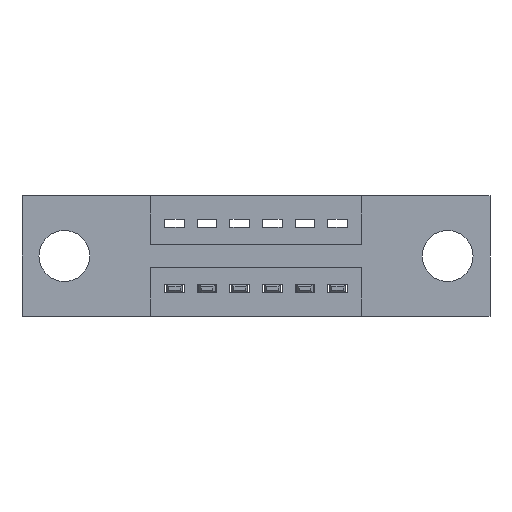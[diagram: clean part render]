
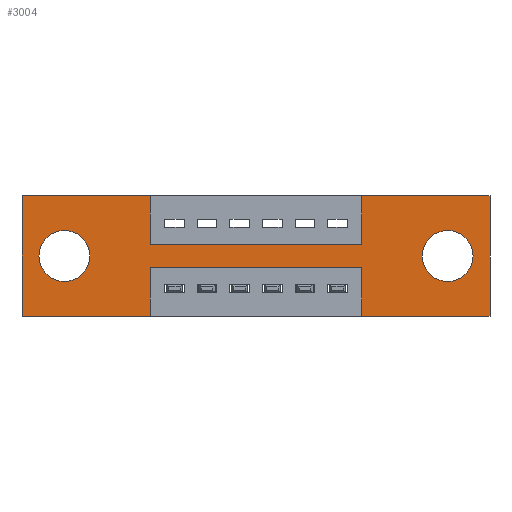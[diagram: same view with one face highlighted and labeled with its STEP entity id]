
A CAD part, front view. The second image highlights one B-rep face of the part: STEP entity #3004.
In plain terms, the highlighted planar face has unit normal (0, -1, 0).
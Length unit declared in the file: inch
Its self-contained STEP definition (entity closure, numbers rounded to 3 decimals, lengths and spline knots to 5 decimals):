
#263 = LINE ( 'NONE', #8894, #2155 ) ;
#273 = CARTESIAN_POINT ( 'NONE',  ( 0.13, 0., -0.185 ) ) ;
#449 = ORIENTED_EDGE ( 'NONE', *, *, #6010, .F. ) ;
#510 = ORIENTED_EDGE ( 'NONE', *, *, #3561, .F. ) ;
#656 = CARTESIAN_POINT ( 'NONE',  ( 0., 0., -0.37 ) ) ;
#702 = DIRECTION ( 'NONE',  ( 0., 0., 1. ) ) ;
#731 = CARTESIAN_POINT ( 'NONE',  ( 1.305, 0., -0.185 ) ) ;
#839 = AXIS2_PLACEMENT_3D ( 'NONE', #273, #4468, #7327 ) ;
#917 = EDGE_CURVE ( 'NONE', #7012, #8329, #1780, .T. ) ;
#924 = LINE ( 'NONE', #656, #3351 ) ;
#969 = FACE_BOUND ( 'NONE', #3698, .T. ) ;
#1025 = ORIENTED_EDGE ( 'NONE', *, *, #6048, .F. ) ;
#1088 = VECTOR ( 'NONE', #5413, 39.37008 ) ;
#1131 = ORIENTED_EDGE ( 'NONE', *, *, #6617, .F. ) ;
#1384 = CARTESIAN_POINT ( 'NONE',  ( 0.3925, 0., -0.22 ) ) ;
#1417 = EDGE_CURVE ( 'NONE', #2836, #5305, #6530, .T. ) ;
#1421 = LINE ( 'NONE', #6382, #8952 ) ;
#1458 = DIRECTION ( 'NONE',  ( -1., 0., 0. ) ) ;
#1647 = CARTESIAN_POINT ( 'NONE',  ( 0.13, 0., -0.263 ) ) ;
#1678 = EDGE_CURVE ( 'NONE', #3209, #7012, #3873, .T. ) ;
#1683 = AXIS2_PLACEMENT_3D ( 'NONE', #5897, #7960, #3851 ) ;
#1780 = LINE ( 'NONE', #1913, #9081 ) ;
#1822 = EDGE_CURVE ( 'NONE', #7105, #2836, #8498, .T. ) ;
#1888 = AXIS2_PLACEMENT_3D ( 'NONE', #3961, #8211, #2530 ) ;
#1913 = CARTESIAN_POINT ( 'NONE',  ( 0.3925, 0., -0.37 ) ) ;
#1924 = AXIS2_PLACEMENT_3D ( 'NONE', #731, #2257, #4273 ) ;
#1944 = VECTOR ( 'NONE', #5935, 39.37008 ) ;
#1992 = EDGE_CURVE ( 'NONE', #6641, #8614, #2429, .T. ) ;
#1994 = CIRCLE ( 'NONE', #1888, 0.078 ) ;
#2011 = CARTESIAN_POINT ( 'NONE',  ( 0., 0., 0. ) ) ;
#2080 = DIRECTION ( 'NONE',  ( 0., 0., 1. ) ) ;
#2155 = VECTOR ( 'NONE', #5618, 39.37008 ) ;
#2207 = CARTESIAN_POINT ( 'NONE',  ( 1.0425, 0., -0.15 ) ) ;
#2257 = DIRECTION ( 'NONE',  ( 0., 1., 0. ) ) ;
#2269 = ORIENTED_EDGE ( 'NONE', *, *, #5813, .T. ) ;
#2362 = ORIENTED_EDGE ( 'NONE', *, *, #7032, .T. ) ;
#2400 = ORIENTED_EDGE ( 'NONE', *, *, #1678, .F. ) ;
#2429 = LINE ( 'NONE', #4110, #9052 ) ;
#2519 = CARTESIAN_POINT ( 'NONE',  ( 1.435, 0., 0. ) ) ;
#2530 = DIRECTION ( 'NONE',  ( 0., 0., -1. ) ) ;
#2575 = VERTEX_POINT ( 'NONE', #5011 ) ;
#2611 = VECTOR ( 'NONE', #8573, 39.37008 ) ;
#2644 = DIRECTION ( 'NONE',  ( 0., 0., -1. ) ) ;
#2649 = EDGE_CURVE ( 'NONE', #3778, #6943, #4633, .T. ) ;
#2684 = EDGE_LOOP ( 'NONE', ( #4541, #2362 ) ) ;
#2734 = DIRECTION ( 'NONE',  ( -1., 0., 0. ) ) ;
#2836 = VERTEX_POINT ( 'NONE', #7200 ) ;
#2890 = CARTESIAN_POINT ( 'NONE',  ( 0., 0., 0. ) ) ;
#2916 = VERTEX_POINT ( 'NONE', #3874 ) ;
#2931 = VERTEX_POINT ( 'NONE', #7302 ) ;
#2967 = EDGE_LOOP ( 'NONE', ( #9012, #2400, #6961, #1025, #6428, #6770, #449, #8671, #7054, #510, #5293, #1131 ) ) ;
#2971 = EDGE_CURVE ( 'NONE', #2931, #7101, #3755, .T. ) ;
#3004 = ADVANCED_FACE ( 'NONE', ( #969, #5977, #8613 ), #8026, .T. ) ;
#3106 = CARTESIAN_POINT ( 'NONE',  ( 0., 0., -0.37 ) ) ;
#3209 = VERTEX_POINT ( 'NONE', #5916 ) ;
#3249 = CARTESIAN_POINT ( 'NONE',  ( 0., 0., 0. ) ) ;
#3351 = VECTOR ( 'NONE', #1458, 39.37008 ) ;
#3402 = VECTOR ( 'NONE', #8855, 39.37008 ) ;
#3561 = EDGE_CURVE ( 'NONE', #6943, #4788, #4296, .T. ) ;
#3698 = EDGE_LOOP ( 'NONE', ( #2269, #8166 ) ) ;
#3734 = CARTESIAN_POINT ( 'NONE',  ( 0., 0., 0. ) ) ;
#3755 = CIRCLE ( 'NONE', #839, 0.078 ) ;
#3778 = VERTEX_POINT ( 'NONE', #3106 ) ;
#3807 = CARTESIAN_POINT ( 'NONE',  ( 1.0425, 0., -0.37 ) ) ;
#3823 = EDGE_CURVE ( 'NONE', #4788, #6641, #6928, .T. ) ;
#3851 = DIRECTION ( 'NONE',  ( 0., 0., -1. ) ) ;
#3873 = LINE ( 'NONE', #5941, #3402 ) ;
#3874 = CARTESIAN_POINT ( 'NONE',  ( 1.305, 0., -0.107 ) ) ;
#3961 = CARTESIAN_POINT ( 'NONE',  ( 1.305, 0., -0.185 ) ) ;
#4110 = CARTESIAN_POINT ( 'NONE',  ( 0.3925, 0., -0.15 ) ) ;
#4216 = DIRECTION ( 'NONE',  ( 1., 0., 0. ) ) ;
#4273 = DIRECTION ( 'NONE',  ( 0., 0., -1. ) ) ;
#4296 = LINE ( 'NONE', #3734, #8361 ) ;
#4468 = DIRECTION ( 'NONE',  ( 0., 1., 0. ) ) ;
#4514 = CARTESIAN_POINT ( 'NONE',  ( 0.3925, 0., 0. ) ) ;
#4541 = ORIENTED_EDGE ( 'NONE', *, *, #2971, .T. ) ;
#4633 = LINE ( 'NONE', #2890, #2611 ) ;
#4710 = DIRECTION ( 'NONE',  ( 1., 0., 0. ) ) ;
#4788 = VERTEX_POINT ( 'NONE', #7256 ) ;
#5011 = CARTESIAN_POINT ( 'NONE',  ( 1.305, 0., -0.263 ) ) ;
#5250 = CIRCLE ( 'NONE', #8087, 0.078 ) ;
#5293 = ORIENTED_EDGE ( 'NONE', *, *, #2649, .F. ) ;
#5305 = VERTEX_POINT ( 'NONE', #7739 ) ;
#5310 = CARTESIAN_POINT ( 'NONE',  ( 0., 0., -0.37 ) ) ;
#5322 = CARTESIAN_POINT ( 'NONE',  ( 0.3925, 0., -0.37 ) ) ;
#5413 = DIRECTION ( 'NONE',  ( 0., 0., -1. ) ) ;
#5618 = DIRECTION ( 'NONE',  ( 0., 0., 1. ) ) ;
#5683 = DIRECTION ( 'NONE',  ( 0., 1., 0. ) ) ;
#5798 = VECTOR ( 'NONE', #2734, 39.37008 ) ;
#5813 = EDGE_CURVE ( 'NONE', #2916, #2575, #8559, .T. ) ;
#5897 = CARTESIAN_POINT ( 'NONE',  ( 0., 0., -0.37 ) ) ;
#5916 = CARTESIAN_POINT ( 'NONE',  ( 1.0425, 0., -0.22 ) ) ;
#5935 = DIRECTION ( 'NONE',  ( 0., 0., -1. ) ) ;
#5941 = CARTESIAN_POINT ( 'NONE',  ( 0.3925, 0., -0.22 ) ) ;
#5977 = FACE_BOUND ( 'NONE', #2684, .T. ) ;
#6010 = EDGE_CURVE ( 'NONE', #8614, #7105, #263, .T. ) ;
#6048 = EDGE_CURVE ( 'NONE', #5305, #9034, #924, .T. ) ;
#6322 = CARTESIAN_POINT ( 'NONE',  ( 0.13, 0., -0.185 ) ) ;
#6382 = CARTESIAN_POINT ( 'NONE',  ( 1.0425, 0., -0.37 ) ) ;
#6428 = ORIENTED_EDGE ( 'NONE', *, *, #1417, .F. ) ;
#6514 = CARTESIAN_POINT ( 'NONE',  ( 1.0425, 0., 0. ) ) ;
#6530 = LINE ( 'NONE', #2519, #1088 ) ;
#6551 = DIRECTION ( 'NONE',  ( 1., 0., 0. ) ) ;
#6617 = EDGE_CURVE ( 'NONE', #8329, #3778, #8429, .T. ) ;
#6641 = VERTEX_POINT ( 'NONE', #8870 ) ;
#6770 = ORIENTED_EDGE ( 'NONE', *, *, #1822, .F. ) ;
#6928 = LINE ( 'NONE', #4514, #1944 ) ;
#6943 = VERTEX_POINT ( 'NONE', #2011 ) ;
#6961 = ORIENTED_EDGE ( 'NONE', *, *, #8519, .F. ) ;
#7012 = VERTEX_POINT ( 'NONE', #1384 ) ;
#7032 = EDGE_CURVE ( 'NONE', #7101, #2931, #5250, .T. ) ;
#7054 = ORIENTED_EDGE ( 'NONE', *, *, #3823, .F. ) ;
#7101 = VERTEX_POINT ( 'NONE', #1647 ) ;
#7105 = VERTEX_POINT ( 'NONE', #6514 ) ;
#7200 = CARTESIAN_POINT ( 'NONE',  ( 1.435, 0., 0. ) ) ;
#7256 = CARTESIAN_POINT ( 'NONE',  ( 0.3925, 0., 0. ) ) ;
#7302 = CARTESIAN_POINT ( 'NONE',  ( 0.13, 0., -0.107 ) ) ;
#7327 = DIRECTION ( 'NONE',  ( 0., 0., 1. ) ) ;
#7396 = EDGE_CURVE ( 'NONE', #2575, #2916, #1994, .T. ) ;
#7739 = CARTESIAN_POINT ( 'NONE',  ( 1.435, 0., -0.37 ) ) ;
#7934 = VECTOR ( 'NONE', #4710, 39.37008 ) ;
#7960 = DIRECTION ( 'NONE',  ( 0., -1., 0. ) ) ;
#8026 = PLANE ( 'NONE',  #1683 ) ;
#8087 = AXIS2_PLACEMENT_3D ( 'NONE', #6322, #5683, #2080 ) ;
#8166 = ORIENTED_EDGE ( 'NONE', *, *, #7396, .T. ) ;
#8211 = DIRECTION ( 'NONE',  ( 0., 1., 0. ) ) ;
#8329 = VERTEX_POINT ( 'NONE', #5322 ) ;
#8361 = VECTOR ( 'NONE', #6551, 39.37008 ) ;
#8429 = LINE ( 'NONE', #5310, #5798 ) ;
#8498 = LINE ( 'NONE', #3249, #7934 ) ;
#8519 = EDGE_CURVE ( 'NONE', #9034, #3209, #1421, .T. ) ;
#8559 = CIRCLE ( 'NONE', #1924, 0.078 ) ;
#8573 = DIRECTION ( 'NONE',  ( 0., 0., 1. ) ) ;
#8613 = FACE_OUTER_BOUND ( 'NONE', #2967, .T. ) ;
#8614 = VERTEX_POINT ( 'NONE', #2207 ) ;
#8671 = ORIENTED_EDGE ( 'NONE', *, *, #1992, .F. ) ;
#8855 = DIRECTION ( 'NONE',  ( -1., 0., 0. ) ) ;
#8870 = CARTESIAN_POINT ( 'NONE',  ( 0.3925, 0., -0.15 ) ) ;
#8894 = CARTESIAN_POINT ( 'NONE',  ( 1.0425, 0., 0. ) ) ;
#8952 = VECTOR ( 'NONE', #702, 39.37008 ) ;
#9012 = ORIENTED_EDGE ( 'NONE', *, *, #917, .F. ) ;
#9034 = VERTEX_POINT ( 'NONE', #3807 ) ;
#9052 = VECTOR ( 'NONE', #4216, 39.37008 ) ;
#9081 = VECTOR ( 'NONE', #2644, 39.37008 ) ;
